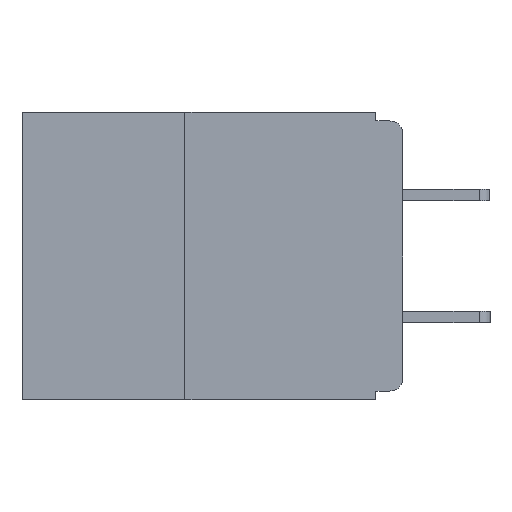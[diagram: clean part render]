
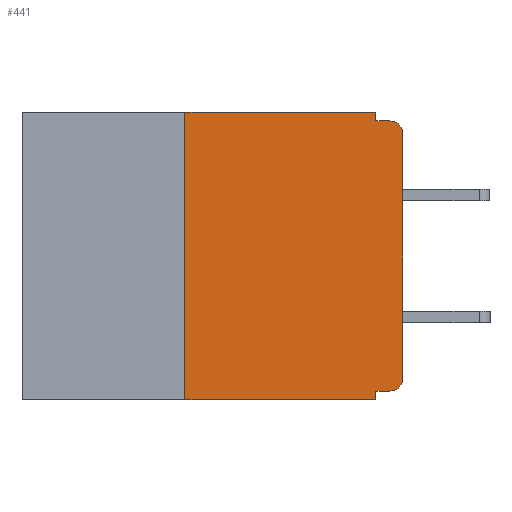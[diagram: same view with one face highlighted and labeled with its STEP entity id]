
A CAD part, left-side view. The second image highlights one B-rep face of the part: STEP entity #441.
In plain terms, the highlighted planar face has unit normal (-1, 0, 0).
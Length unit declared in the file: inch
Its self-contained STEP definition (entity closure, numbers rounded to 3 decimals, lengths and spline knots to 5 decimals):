
#41 = LINE ( 'NONE', #5458, #5998 ) ;
#57 = AXIS2_PLACEMENT_3D ( 'NONE', #168, #13876, #14066 ) ;
#168 = CARTESIAN_POINT ( 'NONE',  ( 0., 0.015, -0.025 ) ) ;
#249 = PLANE ( 'NONE',  #1442 ) ;
#441 = ADVANCED_FACE ( 'NONE', ( #10703 ), #249, .F. ) ;
#649 = EDGE_CURVE ( 'NONE', #4428, #12678, #13831, .T. ) ;
#686 = LINE ( 'NONE', #12929, #11745 ) ;
#794 = EDGE_CURVE ( 'NONE', #12678, #7546, #686, .T. ) ;
#1119 = EDGE_CURVE ( 'NONE', #9866, #14326, #13820, .T. ) ;
#1206 = CARTESIAN_POINT ( 'NONE',  ( 0., 0.031, 0. ) ) ;
#1408 = EDGE_LOOP ( 'NONE', ( #5110, #12660, #10871, #3675, #3524, #14214, #11676, #10050, #8510, #12450 ) ) ;
#1442 = AXIS2_PLACEMENT_3D ( 'NONE', #11602, #8695, #4867 ) ;
#1663 = VERTEX_POINT ( 'NONE', #6766 ) ;
#1797 = DIRECTION ( 'NONE',  ( 0., 0., 1. ) ) ;
#1958 = EDGE_CURVE ( 'NONE', #14326, #7254, #5729, .T. ) ;
#1988 = EDGE_CURVE ( 'NONE', #4428, #9866, #11166, .T. ) ;
#2362 = EDGE_CURVE ( 'NONE', #10584, #7546, #6069, .T. ) ;
#2497 = CARTESIAN_POINT ( 'NONE',  ( 0., 0., 0. ) ) ;
#3121 = CARTESIAN_POINT ( 'NONE',  ( 0., 0., -0.32 ) ) ;
#3127 = DIRECTION ( 'NONE',  ( 0., 1., 0. ) ) ;
#3444 = VERTEX_POINT ( 'NONE', #1206 ) ;
#3524 = ORIENTED_EDGE ( 'NONE', *, *, #8558, .F. ) ;
#3572 = CARTESIAN_POINT ( 'NONE',  ( 0., 0., -0.305 ) ) ;
#3675 = ORIENTED_EDGE ( 'NONE', *, *, #11688, .F. ) ;
#3679 = CARTESIAN_POINT ( 'NONE',  ( 0., 0.031, 0. ) ) ;
#3985 = CARTESIAN_POINT ( 'NONE',  ( 0., 0.031, -0.33 ) ) ;
#4428 = VERTEX_POINT ( 'NONE', #14110 ) ;
#4588 = LINE ( 'NONE', #5802, #10049 ) ;
#4867 = DIRECTION ( 'NONE',  ( 0., 0., -1. ) ) ;
#5110 = ORIENTED_EDGE ( 'NONE', *, *, #1119, .T. ) ;
#5172 = CARTESIAN_POINT ( 'NONE',  ( 0., 0.437, -0.33 ) ) ;
#5458 = CARTESIAN_POINT ( 'NONE',  ( 0., 0.25, -0.33 ) ) ;
#5711 = DIRECTION ( 'NONE',  ( 0., -1., 0. ) ) ;
#5729 = CIRCLE ( 'NONE', #57, 0.015 ) ;
#5802 = CARTESIAN_POINT ( 'NONE',  ( 0., 0.437, 0. ) ) ;
#5998 = VECTOR ( 'NONE', #6584, 39.37008 ) ;
#6069 = LINE ( 'NONE', #5172, #11873 ) ;
#6220 = LINE ( 'NONE', #3679, #8759 ) ;
#6558 = LINE ( 'NONE', #6633, #14257 ) ;
#6584 = DIRECTION ( 'NONE',  ( 0., 0., 1. ) ) ;
#6633 = CARTESIAN_POINT ( 'NONE',  ( 0., 0., -0.01 ) ) ;
#6766 = CARTESIAN_POINT ( 'NONE',  ( 0., 0.25, 0. ) ) ;
#6814 = AXIS2_PLACEMENT_3D ( 'NONE', #13512, #6924, #12431 ) ;
#6924 = DIRECTION ( 'NONE',  ( -1., 0., 0. ) ) ;
#6940 = DIRECTION ( 'NONE',  ( 0., -1., 0. ) ) ;
#7254 = VERTEX_POINT ( 'NONE', #11151 ) ;
#7412 = CARTESIAN_POINT ( 'NONE',  ( 0., 0., -0.025 ) ) ;
#7546 = VERTEX_POINT ( 'NONE', #3985 ) ;
#8191 = CARTESIAN_POINT ( 'NONE',  ( 0., 0.25, -0.33 ) ) ;
#8510 = ORIENTED_EDGE ( 'NONE', *, *, #649, .F. ) ;
#8511 = CARTESIAN_POINT ( 'NONE',  ( 0., 0.031, -0.01 ) ) ;
#8558 = EDGE_CURVE ( 'NONE', #1663, #3444, #4588, .T. ) ;
#8695 = DIRECTION ( 'NONE',  ( 1., 0., 0. ) ) ;
#8759 = VECTOR ( 'NONE', #10229, 39.37008 ) ;
#8918 = CARTESIAN_POINT ( 'NONE',  ( 0., 0.031, -0.32 ) ) ;
#8950 = DIRECTION ( 'NONE',  ( 0., 0., -1. ) ) ;
#9866 = VERTEX_POINT ( 'NONE', #3572 ) ;
#10049 = VECTOR ( 'NONE', #6940, 39.37008 ) ;
#10050 = ORIENTED_EDGE ( 'NONE', *, *, #794, .F. ) ;
#10229 = DIRECTION ( 'NONE',  ( 0., 0., -1. ) ) ;
#10584 = VERTEX_POINT ( 'NONE', #8191 ) ;
#10703 = FACE_OUTER_BOUND ( 'NONE', #1408, .T. ) ;
#10758 = VERTEX_POINT ( 'NONE', #8511 ) ;
#10850 = VECTOR ( 'NONE', #1797, 39.37008 ) ;
#10862 = VECTOR ( 'NONE', #3127, 39.37008 ) ;
#10871 = ORIENTED_EDGE ( 'NONE', *, *, #12168, .F. ) ;
#10972 = DIRECTION ( 'NONE',  ( 0., -1., 0. ) ) ;
#11151 = CARTESIAN_POINT ( 'NONE',  ( 0., 0.015, -0.01 ) ) ;
#11166 = CIRCLE ( 'NONE', #6814, 0.015 ) ;
#11602 = CARTESIAN_POINT ( 'NONE',  ( 0., 0.437, 0. ) ) ;
#11676 = ORIENTED_EDGE ( 'NONE', *, *, #2362, .T. ) ;
#11688 = EDGE_CURVE ( 'NONE', #3444, #10758, #6220, .T. ) ;
#11745 = VECTOR ( 'NONE', #8950, 39.37008 ) ;
#11873 = VECTOR ( 'NONE', #5711, 39.37008 ) ;
#12168 = EDGE_CURVE ( 'NONE', #10758, #7254, #6558, .T. ) ;
#12431 = DIRECTION ( 'NONE',  ( 0., 0., -1. ) ) ;
#12450 = ORIENTED_EDGE ( 'NONE', *, *, #1988, .T. ) ;
#12660 = ORIENTED_EDGE ( 'NONE', *, *, #1958, .T. ) ;
#12678 = VERTEX_POINT ( 'NONE', #8918 ) ;
#12929 = CARTESIAN_POINT ( 'NONE',  ( 0., 0.031, -0.33 ) ) ;
#13512 = CARTESIAN_POINT ( 'NONE',  ( 0., 0.015, -0.305 ) ) ;
#13820 = LINE ( 'NONE', #2497, #10850 ) ;
#13831 = LINE ( 'NONE', #3121, #10862 ) ;
#13834 = EDGE_CURVE ( 'NONE', #10584, #1663, #41, .T. ) ;
#13876 = DIRECTION ( 'NONE',  ( -1., 0., 0. ) ) ;
#14066 = DIRECTION ( 'NONE',  ( 0., 0., -1. ) ) ;
#14110 = CARTESIAN_POINT ( 'NONE',  ( 0., 0.015, -0.32 ) ) ;
#14214 = ORIENTED_EDGE ( 'NONE', *, *, #13834, .F. ) ;
#14257 = VECTOR ( 'NONE', #10972, 39.37008 ) ;
#14326 = VERTEX_POINT ( 'NONE', #7412 ) ;
